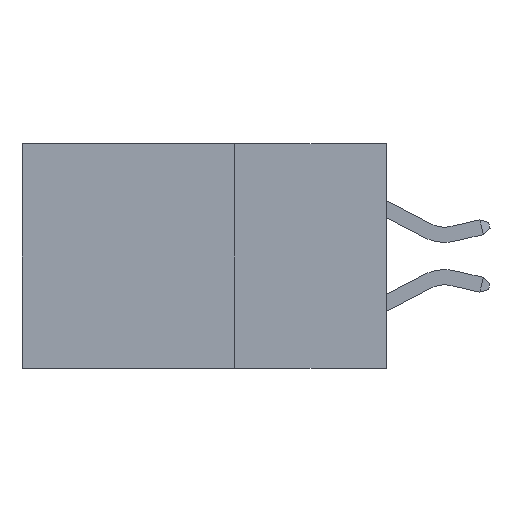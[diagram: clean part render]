
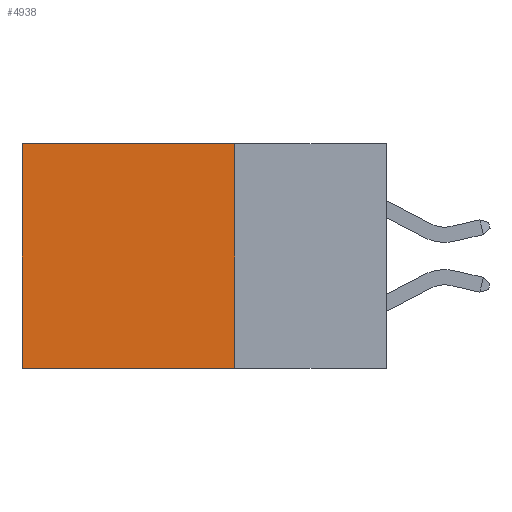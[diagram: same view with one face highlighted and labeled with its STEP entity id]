
A CAD part, left-side view. The second image highlights one B-rep face of the part: STEP entity #4938.
In plain terms, the highlighted planar face has unit normal (-1, 0, 0).
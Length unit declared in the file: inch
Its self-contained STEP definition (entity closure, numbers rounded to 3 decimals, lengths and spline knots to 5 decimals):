
#1013 = CARTESIAN_POINT ( 'NONE',  ( 0.2615, 0.6, 0. ) ) ;
#2374 = CARTESIAN_POINT ( 'NONE',  ( 0.2615, 0.25, 0. ) ) ;
#3886 = CARTESIAN_POINT ( 'NONE',  ( 0.2615, 0.25, -0.37 ) ) ;
#3979 = DIRECTION ( 'NONE',  ( 0., 0., -1. ) ) ;
#4100 = EDGE_CURVE ( 'NONE', #12891, #7049, #5276, .T. ) ;
#4415 = VECTOR ( 'NONE', #13676, 39.37008 ) ;
#4938 = ADVANCED_FACE ( 'NONE', ( #7893 ), #15329, .F. ) ;
#5276 = LINE ( 'NONE', #6567, #6500 ) ;
#5637 = CARTESIAN_POINT ( 'NONE',  ( 0.2615, 0.25, -0.37 ) ) ;
#5917 = DIRECTION ( 'NONE',  ( 0., 1., 0. ) ) ;
#5925 = VERTEX_POINT ( 'NONE', #9474 ) ;
#6161 = EDGE_CURVE ( 'NONE', #8455, #5925, #11788, .T. ) ;
#6500 = VECTOR ( 'NONE', #3979, 39.37008 ) ;
#6567 = CARTESIAN_POINT ( 'NONE',  ( 0.2615, 0.25, -0.37 ) ) ;
#7049 = VERTEX_POINT ( 'NONE', #9883 ) ;
#7262 = EDGE_CURVE ( 'NONE', #12891, #8455, #14573, .T. ) ;
#7363 = LINE ( 'NONE', #3886, #4415 ) ;
#7489 = ORIENTED_EDGE ( 'NONE', *, *, #4100, .F. ) ;
#7830 = VECTOR ( 'NONE', #5917, 39.37008 ) ;
#7893 = FACE_OUTER_BOUND ( 'NONE', #9255, .T. ) ;
#8154 = DIRECTION ( 'NONE',  ( 0., 0., -1. ) ) ;
#8428 = ORIENTED_EDGE ( 'NONE', *, *, #7262, .T. ) ;
#8455 = VERTEX_POINT ( 'NONE', #1013 ) ;
#9255 = EDGE_LOOP ( 'NONE', ( #14158, #15910, #7489, #8428 ) ) ;
#9365 = CARTESIAN_POINT ( 'NONE',  ( 0.2615, 0.6, -0.37 ) ) ;
#9474 = CARTESIAN_POINT ( 'NONE',  ( 0.2615, 0.6, -0.37 ) ) ;
#9883 = CARTESIAN_POINT ( 'NONE',  ( 0.2615, 0.25, -0.37 ) ) ;
#10536 = DIRECTION ( 'NONE',  ( 1., 0., 0. ) ) ;
#11788 = LINE ( 'NONE', #9365, #12621 ) ;
#12621 = VECTOR ( 'NONE', #8154, 39.37008 ) ;
#12891 = VERTEX_POINT ( 'NONE', #13130 ) ;
#13130 = CARTESIAN_POINT ( 'NONE',  ( 0.2615, 0.25, 0. ) ) ;
#13525 = EDGE_CURVE ( 'NONE', #7049, #5925, #7363, .T. ) ;
#13676 = DIRECTION ( 'NONE',  ( 0., 1., 0. ) ) ;
#14062 = AXIS2_PLACEMENT_3D ( 'NONE', #5637, #10536, #15406 ) ;
#14158 = ORIENTED_EDGE ( 'NONE', *, *, #6161, .T. ) ;
#14573 = LINE ( 'NONE', #2374, #7830 ) ;
#15329 = PLANE ( 'NONE',  #14062 ) ;
#15406 = DIRECTION ( 'NONE',  ( 0., 0., -1. ) ) ;
#15910 = ORIENTED_EDGE ( 'NONE', *, *, #13525, .F. ) ;
